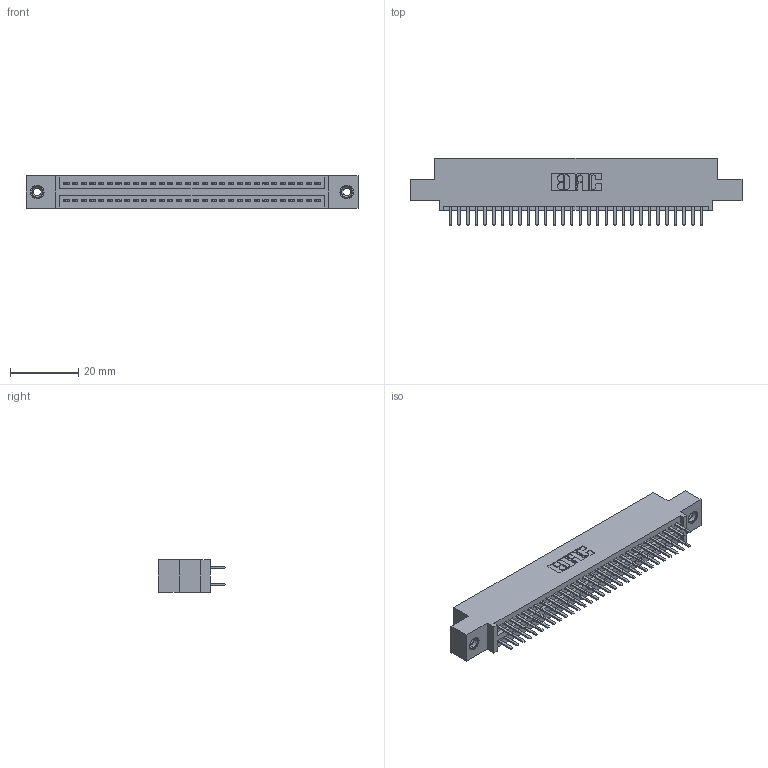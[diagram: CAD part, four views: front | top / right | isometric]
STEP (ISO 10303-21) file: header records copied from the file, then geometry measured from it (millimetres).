
FILE_DESCRIPTION (( 'STEP AP203' ), '1' );
FILE_NAME ('345-060-520-508.STEP', '2019-10-30T07:07:25', ( '' ), ( '' ), 'SwSTEP 2.0', 'SolidWorks 2016', '' );
FILE_SCHEMA (( 'CONFIG_CONTROL_DESIGN' ));
Length unit declared in the file: inch
Products named in the file (4): 345-292-001_345-293-120; 345 Part_0.110 Offset - 0.156 Dia-TI; 345-250-001_345-250-003-102; 345-060-520-508
Assembly tree (63 placements, depth 2):
  345-060-520-508
    345 Part_0.110 Offset - 0.156 Dia-TI
    345-292-001_345-293-120  x60
    345-250-001_345-250-003-102  x2
Bounding box: 97.41 x 19.68 x 9.4 mm (x, y, z)
Volume: 9244.8 mm3; surface area: 13483.1 mm2
Topology: 63 solids, 63 shells, 3430 faces, 9909 edges, 6438 vertices
Faces by surface type: plane 2216, cylinder 1198, cone 12, torus 4
Entity records: 26586 total; most frequent: CARTESIAN_POINT 4463, ORIENTED_EDGE 4378, DIRECTION 3963, EDGE_CURVE 2189, LINE 1913, VECTOR 1913, VERTEX_POINT 1452, AXIS2_PLACEMENT_3D 1025
